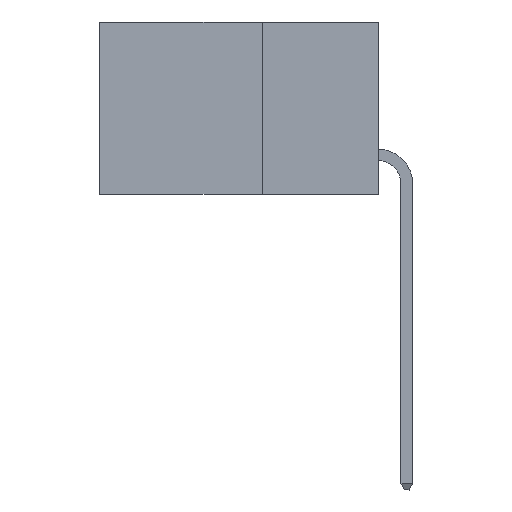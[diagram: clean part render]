
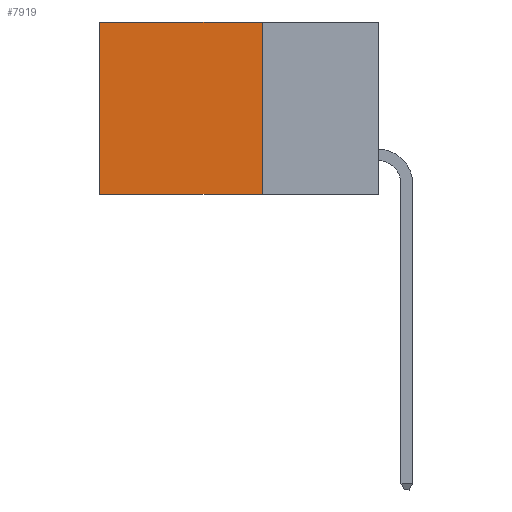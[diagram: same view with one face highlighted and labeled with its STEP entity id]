
A CAD part, left-side view. The second image highlights one B-rep face of the part: STEP entity #7919.
In plain terms, the highlighted planar face has unit normal (-1, 0, 0).
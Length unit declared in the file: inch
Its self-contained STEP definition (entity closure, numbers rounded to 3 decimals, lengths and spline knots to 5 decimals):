
#105 = LINE ( 'NONE', #771, #5171 ) ;
#223 = ORIENTED_EDGE ( 'NONE', *, *, #1329, .F. ) ;
#299 = LINE ( 'NONE', #10149, #10208 ) ;
#683 = DIRECTION ( 'NONE',  ( 0., 0., -1. ) ) ;
#771 = CARTESIAN_POINT ( 'NONE',  ( 0.298, 0.25, 0. ) ) ;
#1124 = EDGE_CURVE ( 'NONE', #2973, #8353, #2355, .T. ) ;
#1329 = EDGE_CURVE ( 'NONE', #11653, #8276, #105, .T. ) ;
#1686 = DIRECTION ( 'NONE',  ( 0., 1., 0. ) ) ;
#2355 = LINE ( 'NONE', #5846, #9623 ) ;
#2747 = FACE_OUTER_BOUND ( 'NONE', #5979, .T. ) ;
#2973 = VERTEX_POINT ( 'NONE', #6264 ) ;
#4413 = CARTESIAN_POINT ( 'NONE',  ( 0.298, 0.6, -0.37 ) ) ;
#4677 = ORIENTED_EDGE ( 'NONE', *, *, #9707, .T. ) ;
#4745 = DIRECTION ( 'NONE',  ( 0., 0., -1. ) ) ;
#5171 = VECTOR ( 'NONE', #4745, 39.37008 ) ;
#5309 = ORIENTED_EDGE ( 'NONE', *, *, #1124, .T. ) ;
#5372 = CARTESIAN_POINT ( 'NONE',  ( 0.298, 0.25, 0. ) ) ;
#5651 = CARTESIAN_POINT ( 'NONE',  ( 0.298, 0.25, 0. ) ) ;
#5846 = CARTESIAN_POINT ( 'NONE',  ( 0.298, 0.6, 0. ) ) ;
#5979 = EDGE_LOOP ( 'NONE', ( #5309, #10337, #223, #4677 ) ) ;
#6264 = CARTESIAN_POINT ( 'NONE',  ( 0.298, 0.6, 0. ) ) ;
#6631 = DIRECTION ( 'NONE',  ( 1., 0., 0. ) ) ;
#6671 = EDGE_CURVE ( 'NONE', #8276, #8353, #299, .T. ) ;
#7123 = VECTOR ( 'NONE', #1686, 39.37008 ) ;
#7400 = LINE ( 'NONE', #5651, #7123 ) ;
#7919 = ADVANCED_FACE ( 'NONE', ( #2747 ), #11977, .F. ) ;
#8049 = AXIS2_PLACEMENT_3D ( 'NONE', #9328, #6631, #683 ) ;
#8276 = VERTEX_POINT ( 'NONE', #8932 ) ;
#8353 = VERTEX_POINT ( 'NONE', #4413 ) ;
#8774 = DIRECTION ( 'NONE',  ( 0., 0., -1. ) ) ;
#8932 = CARTESIAN_POINT ( 'NONE',  ( 0.298, 0.25, -0.37 ) ) ;
#9328 = CARTESIAN_POINT ( 'NONE',  ( 0.298, 0.25, 0. ) ) ;
#9623 = VECTOR ( 'NONE', #8774, 39.37008 ) ;
#9707 = EDGE_CURVE ( 'NONE', #11653, #2973, #7400, .T. ) ;
#10106 = DIRECTION ( 'NONE',  ( 0., 1., 0. ) ) ;
#10149 = CARTESIAN_POINT ( 'NONE',  ( 0.298, 0.25, -0.37 ) ) ;
#10208 = VECTOR ( 'NONE', #10106, 39.37008 ) ;
#10337 = ORIENTED_EDGE ( 'NONE', *, *, #6671, .F. ) ;
#11653 = VERTEX_POINT ( 'NONE', #5372 ) ;
#11977 = PLANE ( 'NONE',  #8049 ) ;
